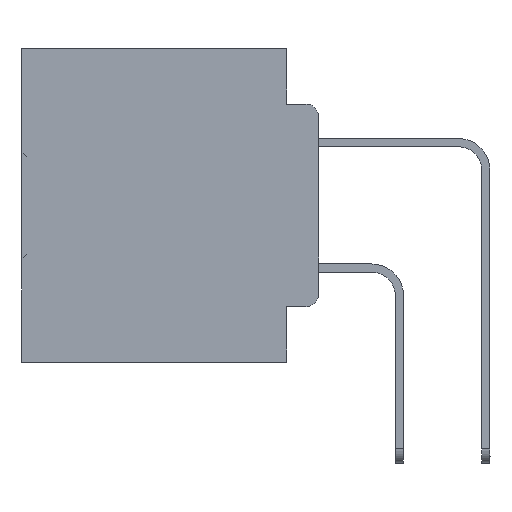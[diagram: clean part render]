
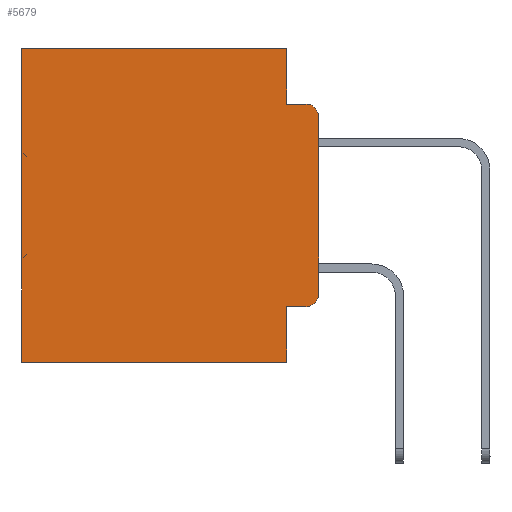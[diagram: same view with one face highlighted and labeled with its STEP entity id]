
A CAD part, left-side view. The second image highlights one B-rep face of the part: STEP entity #5679.
In plain terms, the highlighted planar face has unit normal (-1, 0, 0).
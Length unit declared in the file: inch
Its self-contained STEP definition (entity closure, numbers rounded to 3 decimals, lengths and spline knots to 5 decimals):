
#336 = DIRECTION ( 'NONE',  ( 0., 0., -1. ) ) ;
#526 = CARTESIAN_POINT ( 'NONE',  ( 0.298, 0., 0. ) ) ;
#1101 = EDGE_CURVE ( 'NONE', #28329, #1127, #4981, .T. ) ;
#1127 = VERTEX_POINT ( 'NONE', #22333 ) ;
#1197 = ORIENTED_EDGE ( 'NONE', *, *, #38446, .F. ) ;
#2242 = DIRECTION ( 'NONE',  ( 0., -1., 0. ) ) ;
#2783 = EDGE_CURVE ( 'NONE', #34723, #28329, #20575, .T. ) ;
#3097 = DIRECTION ( 'NONE',  ( 0., -1., 0. ) ) ;
#3490 = DIRECTION ( 'NONE',  ( 0., 0., -1. ) ) ;
#3565 = AXIS2_PLACEMENT_3D ( 'NONE', #12265, #29443, #14810 ) ;
#4625 = CARTESIAN_POINT ( 'NONE',  ( 0.298, 0.051, -0.5 ) ) ;
#4946 = CARTESIAN_POINT ( 'NONE',  ( 0.298, 0., -0.5 ) ) ;
#4981 = LINE ( 'NONE', #31894, #5234 ) ;
#5234 = VECTOR ( 'NONE', #2242, 39.37008 ) ;
#5273 = ORIENTED_EDGE ( 'NONE', *, *, #17136, .F. ) ;
#5328 = VERTEX_POINT ( 'NONE', #19681 ) ;
#5365 = VERTEX_POINT ( 'NONE', #13830 ) ;
#5679 = ADVANCED_FACE ( 'NONE', ( #6181 ), #18046, .F. ) ;
#6181 = FACE_OUTER_BOUND ( 'NONE', #17954, .T. ) ;
#7562 = DIRECTION ( 'NONE',  ( 0., 0., -1. ) ) ;
#8544 = CARTESIAN_POINT ( 'NONE',  ( 0.298, 0.051, -0.0885 ) ) ;
#9519 = CARTESIAN_POINT ( 'NONE',  ( 0.298, 0.051, -0.4115 ) ) ;
#9917 = LINE ( 'NONE', #13215, #26634 ) ;
#9933 = ORIENTED_EDGE ( 'NONE', *, *, #13491, .T. ) ;
#10628 = VERTEX_POINT ( 'NONE', #4625 ) ;
#10794 = LINE ( 'NONE', #4946, #18695 ) ;
#11695 = LINE ( 'NONE', #9519, #12739 ) ;
#12208 = VERTEX_POINT ( 'NONE', #27609 ) ;
#12265 = CARTESIAN_POINT ( 'NONE',  ( 0.298, 0.02, -0.1085 ) ) ;
#12608 = CARTESIAN_POINT ( 'NONE',  ( 0.298, 0.051, -0.4115 ) ) ;
#12739 = VECTOR ( 'NONE', #3097, 39.37008 ) ;
#12924 = VECTOR ( 'NONE', #35055, 39.37008 ) ;
#13215 = CARTESIAN_POINT ( 'NONE',  ( 0.298, 0.051, 0. ) ) ;
#13491 = EDGE_CURVE ( 'NONE', #27216, #12208, #19605, .T. ) ;
#13669 = EDGE_CURVE ( 'NONE', #26908, #10628, #9917, .T. ) ;
#13791 = EDGE_CURVE ( 'NONE', #25757, #5328, #35452, .T. ) ;
#13830 = CARTESIAN_POINT ( 'NONE',  ( 0.298, 0., -0.1085 ) ) ;
#14810 = DIRECTION ( 'NONE',  ( 0., 0., -1. ) ) ;
#14960 = ORIENTED_EDGE ( 'NONE', *, *, #23560, .T. ) ;
#15174 = DIRECTION ( 'NONE',  ( 0., 1., 0. ) ) ;
#15561 = CARTESIAN_POINT ( 'NONE',  ( 0.298, 0.02, -0.3915 ) ) ;
#16468 = VECTOR ( 'NONE', #17648, 39.37008 ) ;
#17083 = DIRECTION ( 'NONE',  ( 0., 0., -1. ) ) ;
#17136 = EDGE_CURVE ( 'NONE', #5365, #12208, #20004, .T. ) ;
#17392 = ORIENTED_EDGE ( 'NONE', *, *, #2783, .F. ) ;
#17648 = DIRECTION ( 'NONE',  ( 0., 0., -1. ) ) ;
#17862 = DIRECTION ( 'NONE',  ( 1., 0., 0. ) ) ;
#17954 = EDGE_LOOP ( 'NONE', ( #5273, #38042, #35251, #17392, #14960, #29065, #1197, #25531, #34156, #9933 ) ) ;
#18046 = PLANE ( 'NONE',  #35301 ) ;
#18695 = VECTOR ( 'NONE', #22674, 39.37008 ) ;
#19605 = CIRCLE ( 'NONE', #33935, 0.02 ) ;
#19681 = CARTESIAN_POINT ( 'NONE',  ( 0.298, 0.473, -0.5 ) ) ;
#20004 = LINE ( 'NONE', #31930, #31951 ) ;
#20575 = LINE ( 'NONE', #23524, #16468 ) ;
#21540 = EDGE_CURVE ( 'NONE', #26908, #27216, #11695, .T. ) ;
#21563 = CARTESIAN_POINT ( 'NONE',  ( 0.298, 0.02, -0.4115 ) ) ;
#22239 = CIRCLE ( 'NONE', #3565, 0.02 ) ;
#22333 = CARTESIAN_POINT ( 'NONE',  ( 0.298, 0.02, -0.0885 ) ) ;
#22674 = DIRECTION ( 'NONE',  ( 0., 1., 0. ) ) ;
#23524 = CARTESIAN_POINT ( 'NONE',  ( 0.298, 0.051, 0. ) ) ;
#23560 = EDGE_CURVE ( 'NONE', #34723, #25757, #32563, .T. ) ;
#23592 = EDGE_CURVE ( 'NONE', #5365, #1127, #22239, .T. ) ;
#23774 = CARTESIAN_POINT ( 'NONE',  ( 0.298, 0., 0. ) ) ;
#23973 = DIRECTION ( 'NONE',  ( -1., 0., 0. ) ) ;
#25531 = ORIENTED_EDGE ( 'NONE', *, *, #13669, .F. ) ;
#25757 = VERTEX_POINT ( 'NONE', #26047 ) ;
#25976 = CARTESIAN_POINT ( 'NONE',  ( 0.298, 0.051, 0. ) ) ;
#26047 = CARTESIAN_POINT ( 'NONE',  ( 0.298, 0.473, 0. ) ) ;
#26634 = VECTOR ( 'NONE', #7562, 39.37008 ) ;
#26908 = VERTEX_POINT ( 'NONE', #12608 ) ;
#27216 = VERTEX_POINT ( 'NONE', #21563 ) ;
#27609 = CARTESIAN_POINT ( 'NONE',  ( 0.298, 0., -0.3915 ) ) ;
#28329 = VERTEX_POINT ( 'NONE', #8544 ) ;
#29065 = ORIENTED_EDGE ( 'NONE', *, *, #13791, .T. ) ;
#29443 = DIRECTION ( 'NONE',  ( -1., 0., 0. ) ) ;
#31894 = CARTESIAN_POINT ( 'NONE',  ( 0.298, 0.051, -0.0885 ) ) ;
#31930 = CARTESIAN_POINT ( 'NONE',  ( 0.298, 0., 0. ) ) ;
#31951 = VECTOR ( 'NONE', #17083, 39.37008 ) ;
#32563 = LINE ( 'NONE', #23774, #35950 ) ;
#33935 = AXIS2_PLACEMENT_3D ( 'NONE', #15561, #23973, #3490 ) ;
#34156 = ORIENTED_EDGE ( 'NONE', *, *, #21540, .T. ) ;
#34723 = VERTEX_POINT ( 'NONE', #25976 ) ;
#35055 = DIRECTION ( 'NONE',  ( 0., 0., -1. ) ) ;
#35251 = ORIENTED_EDGE ( 'NONE', *, *, #1101, .F. ) ;
#35301 = AXIS2_PLACEMENT_3D ( 'NONE', #526, #17862, #336 ) ;
#35452 = LINE ( 'NONE', #38391, #12924 ) ;
#35950 = VECTOR ( 'NONE', #15174, 39.37008 ) ;
#38042 = ORIENTED_EDGE ( 'NONE', *, *, #23592, .T. ) ;
#38391 = CARTESIAN_POINT ( 'NONE',  ( 0.298, 0.473, 0. ) ) ;
#38446 = EDGE_CURVE ( 'NONE', #10628, #5328, #10794, .T. ) ;
